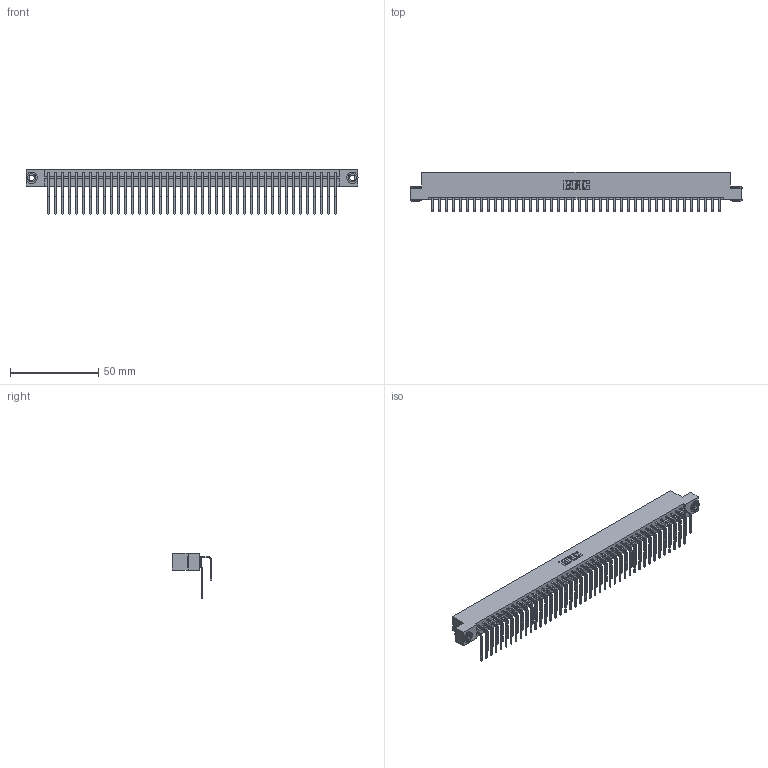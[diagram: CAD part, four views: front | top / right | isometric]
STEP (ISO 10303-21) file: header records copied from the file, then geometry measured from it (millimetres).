
FILE_DESCRIPTION (( 'STEP AP203' ), '1' );
FILE_NAME ('833-084-558-203.STEP', '2020-06-06T02:11:39', ( '' ), ( '' ), 'SwSTEP 2.0', 'SolidWorks 2020', '' );
FILE_SCHEMA (( 'CONFIG_CONTROL_DESIGN' ));
Length unit declared in the file: inch
Products named in the file (5): 345-250-002_345-250-002-102; 833 Part_Flush - .156 Dia - TH; 833-084-558-203; 345-292-001_558 559 Tail - 1; 345-292-001_558 Tail - 2
Assembly tree (87 placements, depth 2):
  833-084-558-203
    833 Part_Flush - .156 Dia - TH
    345-292-001_558 559 Tail - 1  x42
    345-292-001_558 Tail - 2  x42
    345-250-002_345-250-002-102  x2
Bounding box: 187.96 x 22.17 x 25.53 mm (x, y, z)
Volume: 19693.6 mm3; surface area: 25917.3 mm2
Topology: 87 solids, 87 shells, 4688 faces, 13911 edges, 9158 vertices
Faces by surface type: plane 3272, cylinder 1408, cone 8
Entity records: 29454 total; most frequent: CARTESIAN_POINT 4908, ORIENTED_EDGE 4786, DIRECTION 4207, EDGE_CURVE 2393, VECTOR 2201, LINE 2201, VERTEX_POINT 1590, AXIS2_PLACEMENT_3D 1003
